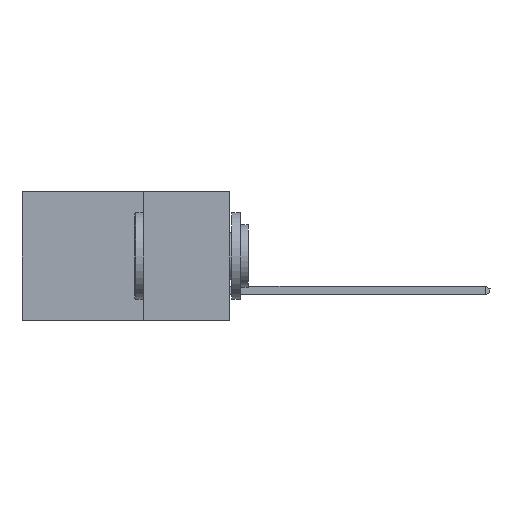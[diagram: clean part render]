
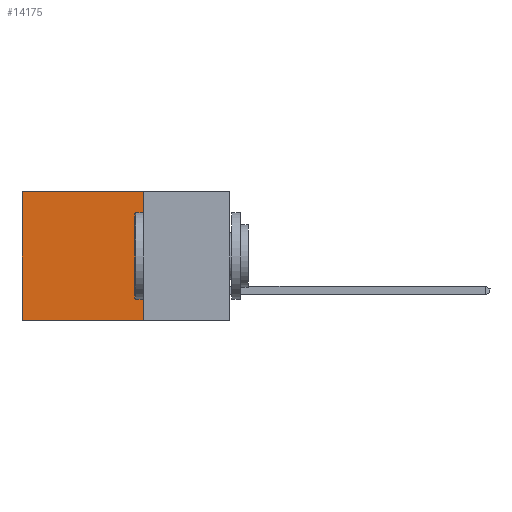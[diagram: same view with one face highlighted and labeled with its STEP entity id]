
A CAD part, left-side view. The second image highlights one B-rep face of the part: STEP entity #14175.
In plain terms, the highlighted planar face has unit normal (-1, 0, 0).
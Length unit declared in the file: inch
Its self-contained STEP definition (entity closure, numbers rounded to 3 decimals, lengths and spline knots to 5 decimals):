
#1528 = EDGE_CURVE ( 'NONE', #11026, #6916, #12336, .T. ) ;
#1589 = LINE ( 'NONE', #7221, #5939 ) ;
#1860 = CARTESIAN_POINT ( 'NONE',  ( 0.2615, 0.25, 0. ) ) ;
#2560 = EDGE_CURVE ( 'NONE', #6916, #5774, #2961, .T. ) ;
#2720 = EDGE_CURVE ( 'NONE', #11026, #12987, #1589, .T. ) ;
#2961 = LINE ( 'NONE', #13513, #3932 ) ;
#3365 = CARTESIAN_POINT ( 'NONE',  ( 0.2615, 0.25, 0. ) ) ;
#3689 = CARTESIAN_POINT ( 'NONE',  ( 0.2615, 0.25, -0.37 ) ) ;
#3932 = VECTOR ( 'NONE', #7777, 39.37008 ) ;
#4559 = DIRECTION ( 'NONE',  ( 1., 0., 0. ) ) ;
#5513 = CARTESIAN_POINT ( 'NONE',  ( 0.2615, 0.25, -0.37 ) ) ;
#5582 = DIRECTION ( 'NONE',  ( 0., 1., 0. ) ) ;
#5774 = VERTEX_POINT ( 'NONE', #11821 ) ;
#5939 = VECTOR ( 'NONE', #14350, 39.37008 ) ;
#6916 = VERTEX_POINT ( 'NONE', #12130 ) ;
#7221 = CARTESIAN_POINT ( 'NONE',  ( 0.2615, 0.25, -0.37 ) ) ;
#7437 = VECTOR ( 'NONE', #5582, 39.37008 ) ;
#7729 = LINE ( 'NONE', #5513, #7437 ) ;
#7777 = DIRECTION ( 'NONE',  ( 0., 0., -1. ) ) ;
#8122 = ORIENTED_EDGE ( 'NONE', *, *, #8916, .F. ) ;
#8487 = DIRECTION ( 'NONE',  ( 0., 1., 0. ) ) ;
#8916 = EDGE_CURVE ( 'NONE', #12987, #5774, #7729, .T. ) ;
#9620 = VECTOR ( 'NONE', #8487, 39.37008 ) ;
#9644 = ORIENTED_EDGE ( 'NONE', *, *, #2560, .T. ) ;
#11026 = VERTEX_POINT ( 'NONE', #3365 ) ;
#11085 = ORIENTED_EDGE ( 'NONE', *, *, #1528, .T. ) ;
#11596 = PLANE ( 'NONE',  #13306 ) ;
#11821 = CARTESIAN_POINT ( 'NONE',  ( 0.2615, 0.6, -0.37 ) ) ;
#12105 = EDGE_LOOP ( 'NONE', ( #9644, #8122, #12301, #11085 ) ) ;
#12130 = CARTESIAN_POINT ( 'NONE',  ( 0.2615, 0.6, 0. ) ) ;
#12301 = ORIENTED_EDGE ( 'NONE', *, *, #2720, .F. ) ;
#12336 = LINE ( 'NONE', #1860, #9620 ) ;
#12915 = DIRECTION ( 'NONE',  ( 0., 0., -1. ) ) ;
#12987 = VERTEX_POINT ( 'NONE', #3689 ) ;
#13306 = AXIS2_PLACEMENT_3D ( 'NONE', #14972, #4559, #12915 ) ;
#13513 = CARTESIAN_POINT ( 'NONE',  ( 0.2615, 0.6, -0.37 ) ) ;
#13557 = FACE_OUTER_BOUND ( 'NONE', #12105, .T. ) ;
#14175 = ADVANCED_FACE ( 'NONE', ( #13557 ), #11596, .F. ) ;
#14350 = DIRECTION ( 'NONE',  ( 0., 0., -1. ) ) ;
#14972 = CARTESIAN_POINT ( 'NONE',  ( 0.2615, 0.25, -0.37 ) ) ;
